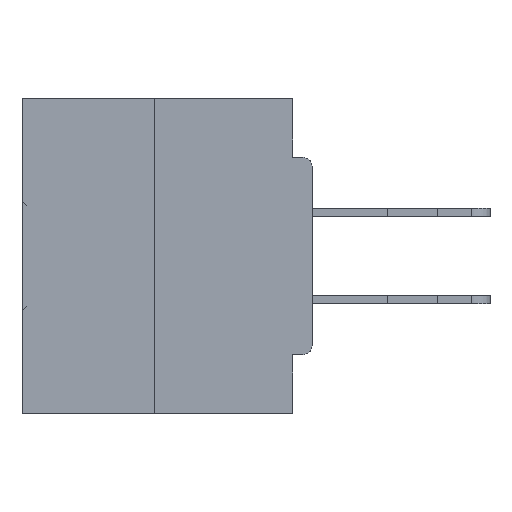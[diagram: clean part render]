
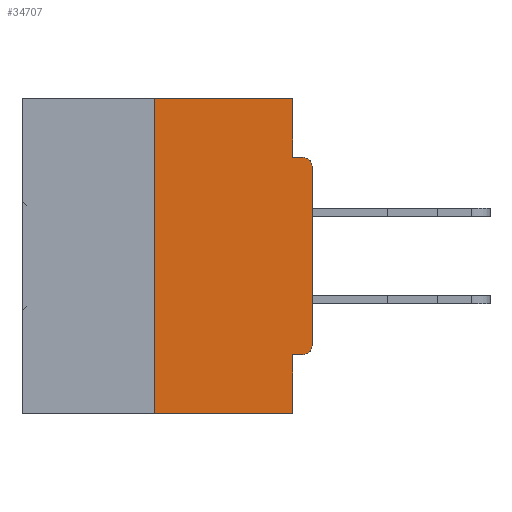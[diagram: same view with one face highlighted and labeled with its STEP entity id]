
A CAD part, left-side view. The second image highlights one B-rep face of the part: STEP entity #34707.
In plain terms, the highlighted planar face has unit normal (-1, 0, 0).
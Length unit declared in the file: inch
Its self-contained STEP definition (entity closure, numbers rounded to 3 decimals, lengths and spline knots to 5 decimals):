
#77 = CARTESIAN_POINT ( 'NONE',  ( 0., 0.015, -0.1085 ) ) ;
#396 = CARTESIAN_POINT ( 'NONE',  ( 0., 0.031, -0.5 ) ) ;
#1526 = CARTESIAN_POINT ( 'NONE',  ( 0., 0.25, 0. ) ) ;
#1554 = VECTOR ( 'NONE', #14205, 39.37008 ) ;
#1680 = LINE ( 'NONE', #39717, #13214 ) ;
#2167 = VERTEX_POINT ( 'NONE', #17684 ) ;
#2701 = VECTOR ( 'NONE', #38240, 39.37008 ) ;
#2750 = VECTOR ( 'NONE', #23602, 39.37008 ) ;
#3802 = LINE ( 'NONE', #27724, #2701 ) ;
#4302 = LINE ( 'NONE', #24839, #1554 ) ;
#4868 = AXIS2_PLACEMENT_3D ( 'NONE', #19501, #23340, #33295 ) ;
#5502 = CARTESIAN_POINT ( 'NONE',  ( 0., 0.46, 0. ) ) ;
#5538 = DIRECTION ( 'NONE',  ( -1., 0., 0. ) ) ;
#5725 = ORIENTED_EDGE ( 'NONE', *, *, #33748, .T. ) ;
#5743 = ORIENTED_EDGE ( 'NONE', *, *, #20213, .F. ) ;
#6096 = VERTEX_POINT ( 'NONE', #396 ) ;
#9078 = EDGE_CURVE ( 'NONE', #33533, #18476, #41838, .T. ) ;
#9195 = DIRECTION ( 'NONE',  ( 0., -1., 0. ) ) ;
#10688 = DIRECTION ( 'NONE',  ( 0., 0., -1. ) ) ;
#10822 = VERTEX_POINT ( 'NONE', #15705 ) ;
#11207 = ORIENTED_EDGE ( 'NONE', *, *, #26253, .T. ) ;
#11244 = VERTEX_POINT ( 'NONE', #38862 ) ;
#11843 = VERTEX_POINT ( 'NONE', #1526 ) ;
#13214 = VECTOR ( 'NONE', #29303, 39.37008 ) ;
#13374 = CARTESIAN_POINT ( 'NONE',  ( 0., 0.031, -0.0935 ) ) ;
#13593 = VECTOR ( 'NONE', #14224, 39.37008 ) ;
#13609 = FACE_OUTER_BOUND ( 'NONE', #28279, .T. ) ;
#14098 = ORIENTED_EDGE ( 'NONE', *, *, #33292, .T. ) ;
#14205 = DIRECTION ( 'NONE',  ( 0., 0., -1. ) ) ;
#14224 = DIRECTION ( 'NONE',  ( 0., 0., 1. ) ) ;
#15299 = CARTESIAN_POINT ( 'NONE',  ( 0., 0.25, 0. ) ) ;
#15655 = ORIENTED_EDGE ( 'NONE', *, *, #24328, .F. ) ;
#15705 = CARTESIAN_POINT ( 'NONE',  ( 0., 0.015, -0.4065 ) ) ;
#17684 = CARTESIAN_POINT ( 'NONE',  ( 0., 0.031, -0.4065 ) ) ;
#17893 = DIRECTION ( 'NONE',  ( -1., 0., 0. ) ) ;
#17996 = LINE ( 'NONE', #28091, #13593 ) ;
#18476 = VERTEX_POINT ( 'NONE', #31057 ) ;
#18928 = ORIENTED_EDGE ( 'NONE', *, *, #23012, .F. ) ;
#19501 = CARTESIAN_POINT ( 'NONE',  ( 0., 0.46, 0. ) ) ;
#20099 = VECTOR ( 'NONE', #9195, 39.37008 ) ;
#20213 = EDGE_CURVE ( 'NONE', #2167, #6096, #1680, .T. ) ;
#20479 = EDGE_CURVE ( 'NONE', #10822, #2167, #26403, .T. ) ;
#21031 = CARTESIAN_POINT ( 'NONE',  ( 0., 0.25, -0.5 ) ) ;
#21092 = VERTEX_POINT ( 'NONE', #13374 ) ;
#21933 = AXIS2_PLACEMENT_3D ( 'NONE', #37280, #5538, #30570 ) ;
#23012 = EDGE_CURVE ( 'NONE', #26297, #21092, #4302, .T. ) ;
#23042 = LINE ( 'NONE', #33178, #32896 ) ;
#23340 = DIRECTION ( 'NONE',  ( 1., 0., 0. ) ) ;
#23446 = DIRECTION ( 'NONE',  ( 0., 0., 1. ) ) ;
#23602 = DIRECTION ( 'NONE',  ( 0., 1., 0. ) ) ;
#24328 = EDGE_CURVE ( 'NONE', #11843, #26297, #34352, .T. ) ;
#24839 = CARTESIAN_POINT ( 'NONE',  ( 0., 0.031, 0. ) ) ;
#26253 = EDGE_CURVE ( 'NONE', #10822, #11244, #45234, .T. ) ;
#26297 = VERTEX_POINT ( 'NONE', #34203 ) ;
#26403 = LINE ( 'NONE', #44605, #2750 ) ;
#27092 = ORIENTED_EDGE ( 'NONE', *, *, #20479, .F. ) ;
#27724 = CARTESIAN_POINT ( 'NONE',  ( 0., 0., -0.0935 ) ) ;
#28091 = CARTESIAN_POINT ( 'NONE',  ( 0., 0., 0. ) ) ;
#28279 = EDGE_LOOP ( 'NONE', ( #15655, #42629, #14098, #5743, #27092, #11207, #5725, #44951, #30581, #18928 ) ) ;
#29303 = DIRECTION ( 'NONE',  ( 0., 0., -1. ) ) ;
#29944 = PLANE ( 'NONE',  #4868 ) ;
#30570 = DIRECTION ( 'NONE',  ( 0., 0., -1. ) ) ;
#30581 = ORIENTED_EDGE ( 'NONE', *, *, #37223, .F. ) ;
#31057 = CARTESIAN_POINT ( 'NONE',  ( 0., 0.015, -0.0935 ) ) ;
#31778 = VERTEX_POINT ( 'NONE', #21031 ) ;
#32140 = VECTOR ( 'NONE', #23446, 39.37008 ) ;
#32896 = VECTOR ( 'NONE', #33488, 39.37008 ) ;
#33178 = CARTESIAN_POINT ( 'NONE',  ( 0., 0.46, -0.5 ) ) ;
#33292 = EDGE_CURVE ( 'NONE', #31778, #6096, #23042, .T. ) ;
#33295 = DIRECTION ( 'NONE',  ( 0., 0., -1. ) ) ;
#33488 = DIRECTION ( 'NONE',  ( 0., -1., 0. ) ) ;
#33533 = VERTEX_POINT ( 'NONE', #45119 ) ;
#33748 = EDGE_CURVE ( 'NONE', #11244, #33533, #17996, .T. ) ;
#34203 = CARTESIAN_POINT ( 'NONE',  ( 0., 0.031, 0. ) ) ;
#34352 = LINE ( 'NONE', #5502, #20099 ) ;
#34707 = ADVANCED_FACE ( 'NONE', ( #13609 ), #29944, .F. ) ;
#37223 = EDGE_CURVE ( 'NONE', #21092, #18476, #3802, .T. ) ;
#37280 = CARTESIAN_POINT ( 'NONE',  ( 0., 0.015, -0.3915 ) ) ;
#38240 = DIRECTION ( 'NONE',  ( 0., -1., 0. ) ) ;
#38862 = CARTESIAN_POINT ( 'NONE',  ( 0., 0., -0.3915 ) ) ;
#39004 = EDGE_CURVE ( 'NONE', #31778, #11843, #41458, .T. ) ;
#39717 = CARTESIAN_POINT ( 'NONE',  ( 0., 0.031, -0.5 ) ) ;
#41458 = LINE ( 'NONE', #15299, #32140 ) ;
#41838 = CIRCLE ( 'NONE', #44759, 0.015 ) ;
#42629 = ORIENTED_EDGE ( 'NONE', *, *, #39004, .F. ) ;
#44605 = CARTESIAN_POINT ( 'NONE',  ( 0., 0., -0.4065 ) ) ;
#44759 = AXIS2_PLACEMENT_3D ( 'NONE', #77, #17893, #10688 ) ;
#44951 = ORIENTED_EDGE ( 'NONE', *, *, #9078, .T. ) ;
#45119 = CARTESIAN_POINT ( 'NONE',  ( 0., 0., -0.1085 ) ) ;
#45234 = CIRCLE ( 'NONE', #21933, 0.015 ) ;
